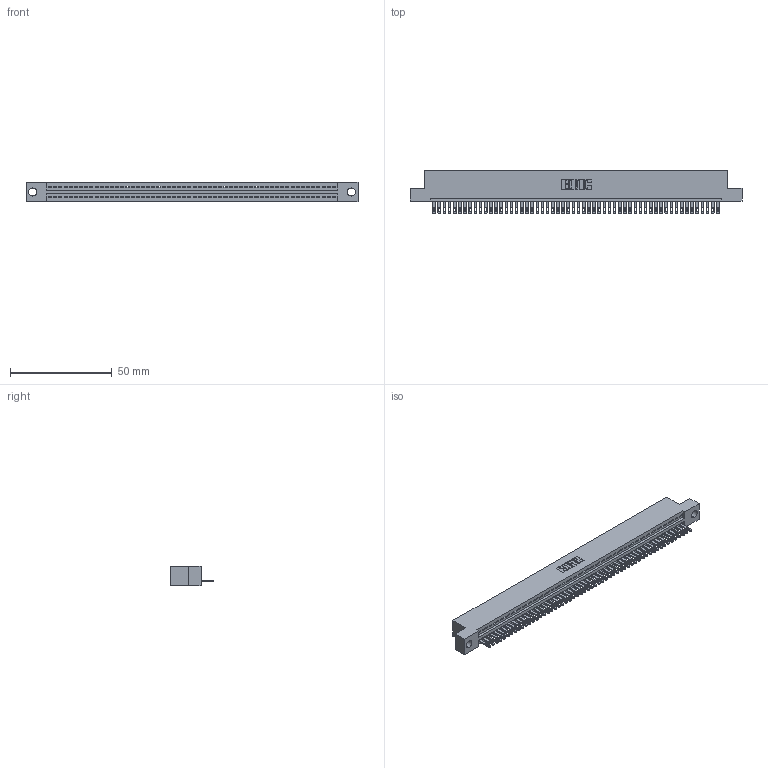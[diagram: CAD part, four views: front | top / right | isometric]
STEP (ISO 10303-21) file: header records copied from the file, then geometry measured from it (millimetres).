
FILE_DESCRIPTION (( 'STEP AP203' ), '1' );
FILE_NAME ('895-056-500-104.STEP', '2020-09-27T15:33:12', ( '' ), ( '' ), 'SwSTEP 2.0', 'SolidWorks 2020', '' );
FILE_SCHEMA (( 'CONFIG_CONTROL_DESIGN' ));
Length unit declared in the file: inch
Products named in the file (3): 345-292-001_345-293-100; 845 Part_Flush Mounting Lugs - 0.156 Dia-TH; 895-056-500-104
Assembly tree (57 placements, depth 2):
  895-056-500-104
    845 Part_Flush Mounting Lugs - 0.156 Dia-TH
    345-292-001_345-293-100  x56
Bounding box: 163.45 x 21.51 x 9.4 mm (x, y, z)
Volume: 15586 mm3; surface area: 20837.2 mm2
Topology: 57 solids, 57 shells, 3150 faces, 9749 edges, 6498 vertices
Faces by surface type: plane 1984, cylinder 1166
Entity records: 40195 total; most frequent: CARTESIAN_POINT 6968, ORIENTED_EDGE 6958, DIRECTION 6067, EDGE_CURVE 3479, VECTOR 3119, LINE 3119, VERTEX_POINT 2318, AXIS2_PLACEMENT_3D 1474
